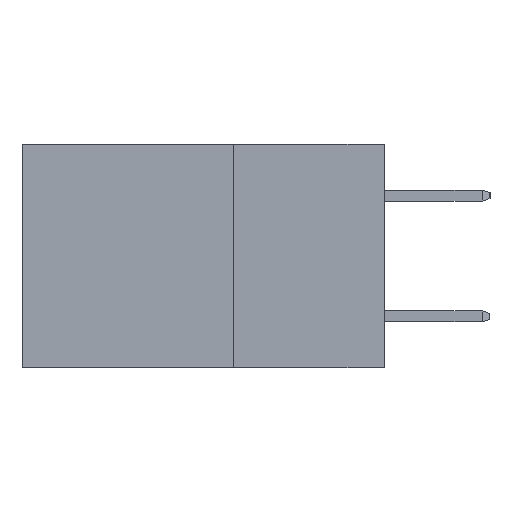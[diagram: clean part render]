
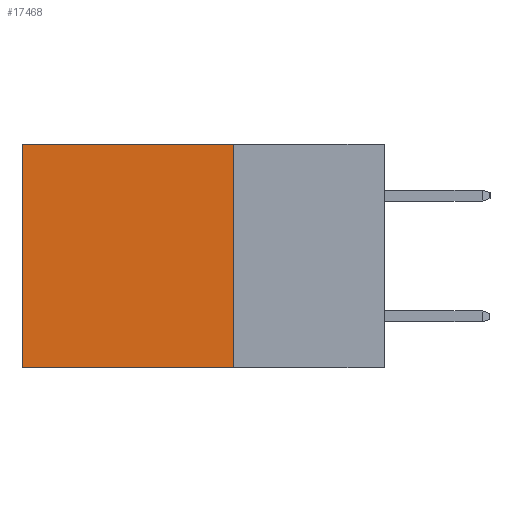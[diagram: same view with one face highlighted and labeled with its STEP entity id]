
A CAD part, left-side view. The second image highlights one B-rep face of the part: STEP entity #17468.
In plain terms, the highlighted planar face has unit normal (-1, 0, 0).
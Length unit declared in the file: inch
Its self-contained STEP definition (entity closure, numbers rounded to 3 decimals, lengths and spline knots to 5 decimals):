
#67 = CARTESIAN_POINT ( 'NONE',  ( 0.298, 0.25, -0.37 ) ) ;
#683 = FACE_OUTER_BOUND ( 'NONE', #15963, .T. ) ;
#993 = AXIS2_PLACEMENT_3D ( 'NONE', #15897, #19006, #9669 ) ;
#1590 = ORIENTED_EDGE ( 'NONE', *, *, #16235, .F. ) ;
#2068 = VECTOR ( 'NONE', #5036, 39.37008 ) ;
#2498 = EDGE_CURVE ( 'NONE', #4206, #18505, #16145, .T. ) ;
#3675 = CARTESIAN_POINT ( 'NONE',  ( 0.298, 0.6, -0.37 ) ) ;
#4206 = VERTEX_POINT ( 'NONE', #18227 ) ;
#5036 = DIRECTION ( 'NONE',  ( 0., 0., -1. ) ) ;
#5564 = VECTOR ( 'NONE', #17213, 39.37008 ) ;
#7193 = DIRECTION ( 'NONE',  ( 0., 1., 0. ) ) ;
#7885 = CARTESIAN_POINT ( 'NONE',  ( 0.298, 0.25, 0. ) ) ;
#8757 = EDGE_CURVE ( 'NONE', #12921, #4206, #13423, .T. ) ;
#8975 = DIRECTION ( 'NONE',  ( 0., 0., -1. ) ) ;
#9284 = CARTESIAN_POINT ( 'NONE',  ( 0.298, 0.6, 0. ) ) ;
#9444 = VECTOR ( 'NONE', #7193, 39.37008 ) ;
#9669 = DIRECTION ( 'NONE',  ( 0., 0., -1. ) ) ;
#10056 = CARTESIAN_POINT ( 'NONE',  ( 0.298, 0.25, 0. ) ) ;
#11027 = EDGE_CURVE ( 'NONE', #12051, #18505, #13589, .T. ) ;
#12051 = VERTEX_POINT ( 'NONE', #67 ) ;
#12851 = CARTESIAN_POINT ( 'NONE',  ( 0.298, 0.25, 0. ) ) ;
#12921 = VERTEX_POINT ( 'NONE', #10056 ) ;
#13423 = LINE ( 'NONE', #7885, #5564 ) ;
#13528 = ORIENTED_EDGE ( 'NONE', *, *, #11027, .F. ) ;
#13589 = LINE ( 'NONE', #18070, #9444 ) ;
#14730 = ORIENTED_EDGE ( 'NONE', *, *, #8757, .T. ) ;
#15897 = CARTESIAN_POINT ( 'NONE',  ( 0.298, 0.25, 0. ) ) ;
#15963 = EDGE_LOOP ( 'NONE', ( #16467, #13528, #1590, #14730 ) ) ;
#16145 = LINE ( 'NONE', #9284, #19754 ) ;
#16235 = EDGE_CURVE ( 'NONE', #12921, #12051, #18757, .T. ) ;
#16467 = ORIENTED_EDGE ( 'NONE', *, *, #2498, .T. ) ;
#17213 = DIRECTION ( 'NONE',  ( 0., 1., 0. ) ) ;
#17450 = PLANE ( 'NONE',  #993 ) ;
#17468 = ADVANCED_FACE ( 'NONE', ( #683 ), #17450, .F. ) ;
#18070 = CARTESIAN_POINT ( 'NONE',  ( 0.298, 0.25, -0.37 ) ) ;
#18227 = CARTESIAN_POINT ( 'NONE',  ( 0.298, 0.6, 0. ) ) ;
#18505 = VERTEX_POINT ( 'NONE', #3675 ) ;
#18757 = LINE ( 'NONE', #12851, #2068 ) ;
#19006 = DIRECTION ( 'NONE',  ( 1., 0., 0. ) ) ;
#19754 = VECTOR ( 'NONE', #8975, 39.37008 ) ;
